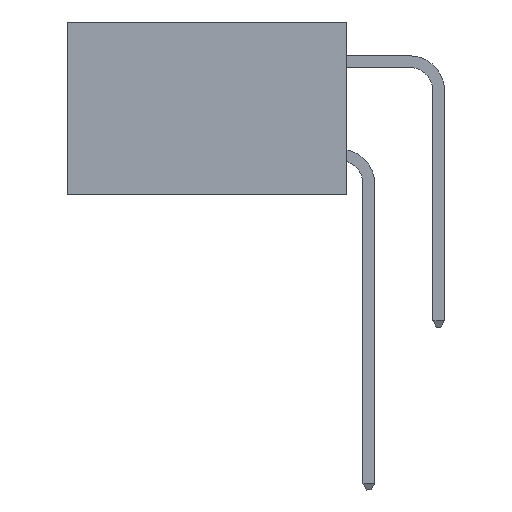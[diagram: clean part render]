
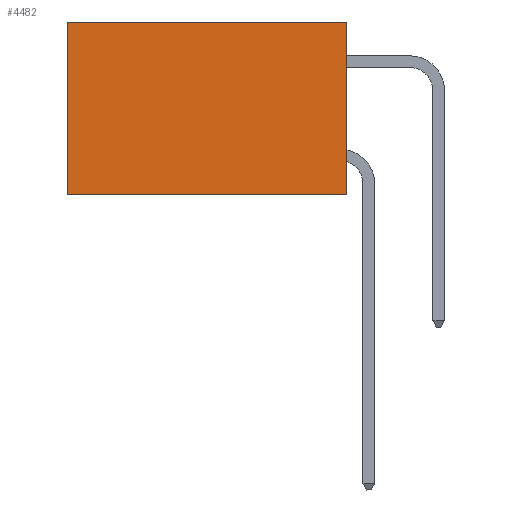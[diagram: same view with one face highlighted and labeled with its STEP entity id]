
A CAD part, left-side view. The second image highlights one B-rep face of the part: STEP entity #4482.
In plain terms, the highlighted planar face has unit normal (-1, 0, 0).
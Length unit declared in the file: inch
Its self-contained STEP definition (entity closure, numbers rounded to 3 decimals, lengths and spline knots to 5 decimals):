
#31 = CARTESIAN_POINT ( 'NONE',  ( 0.2875, 0.6, 0. ) ) ;
#100 = VERTEX_POINT ( 'NONE', #3195 ) ;
#1138 = LINE ( 'NONE', #3362, #14991 ) ;
#2239 = LINE ( 'NONE', #31, #16079 ) ;
#2350 = DIRECTION ( 'NONE',  ( 0., 1., 0. ) ) ;
#2639 = EDGE_CURVE ( 'NONE', #100, #8667, #18511, .T. ) ;
#2774 = DIRECTION ( 'NONE',  ( 0., 0., -1. ) ) ;
#3195 = CARTESIAN_POINT ( 'NONE',  ( 0.2875, 0., -0.37 ) ) ;
#3362 = CARTESIAN_POINT ( 'NONE',  ( 0.2875, 0., 0. ) ) ;
#3828 = VERTEX_POINT ( 'NONE', #17565 ) ;
#3925 = PLANE ( 'NONE',  #10018 ) ;
#4482 = ADVANCED_FACE ( 'NONE', ( #16358 ), #3925, .F. ) ;
#5425 = EDGE_CURVE ( 'NONE', #5940, #100, #1138, .T. ) ;
#5940 = VERTEX_POINT ( 'NONE', #17228 ) ;
#6050 = ORIENTED_EDGE ( 'NONE', *, *, #5425, .F. ) ;
#6634 = ORIENTED_EDGE ( 'NONE', *, *, #13203, .T. ) ;
#6993 = VECTOR ( 'NONE', #10092, 39.37008 ) ;
#7111 = EDGE_CURVE ( 'NONE', #3828, #8667, #2239, .T. ) ;
#8051 = CARTESIAN_POINT ( 'NONE',  ( 0.2875, 0., -0.37 ) ) ;
#8667 = VERTEX_POINT ( 'NONE', #13554 ) ;
#9294 = CARTESIAN_POINT ( 'NONE',  ( 0.2875, 0., 0. ) ) ;
#9409 = ORIENTED_EDGE ( 'NONE', *, *, #2639, .F. ) ;
#10018 = AXIS2_PLACEMENT_3D ( 'NONE', #16706, #15435, #18308 ) ;
#10092 = DIRECTION ( 'NONE',  ( 0., 1., 0. ) ) ;
#11358 = DIRECTION ( 'NONE',  ( 0., 0., -1. ) ) ;
#11671 = ORIENTED_EDGE ( 'NONE', *, *, #7111, .T. ) ;
#11821 = LINE ( 'NONE', #9294, #15937 ) ;
#13203 = EDGE_CURVE ( 'NONE', #5940, #3828, #11821, .T. ) ;
#13554 = CARTESIAN_POINT ( 'NONE',  ( 0.2875, 0.6, -0.37 ) ) ;
#13638 = EDGE_LOOP ( 'NONE', ( #11671, #9409, #6050, #6634 ) ) ;
#14991 = VECTOR ( 'NONE', #11358, 39.37008 ) ;
#15435 = DIRECTION ( 'NONE',  ( 1., 0., 0. ) ) ;
#15937 = VECTOR ( 'NONE', #2350, 39.37008 ) ;
#16079 = VECTOR ( 'NONE', #2774, 39.37008 ) ;
#16358 = FACE_OUTER_BOUND ( 'NONE', #13638, .T. ) ;
#16706 = CARTESIAN_POINT ( 'NONE',  ( 0.2875, 0., 0. ) ) ;
#17228 = CARTESIAN_POINT ( 'NONE',  ( 0.2875, 0., 0. ) ) ;
#17565 = CARTESIAN_POINT ( 'NONE',  ( 0.2875, 0.6, 0. ) ) ;
#18308 = DIRECTION ( 'NONE',  ( 0., 0., -1. ) ) ;
#18511 = LINE ( 'NONE', #8051, #6993 ) ;
